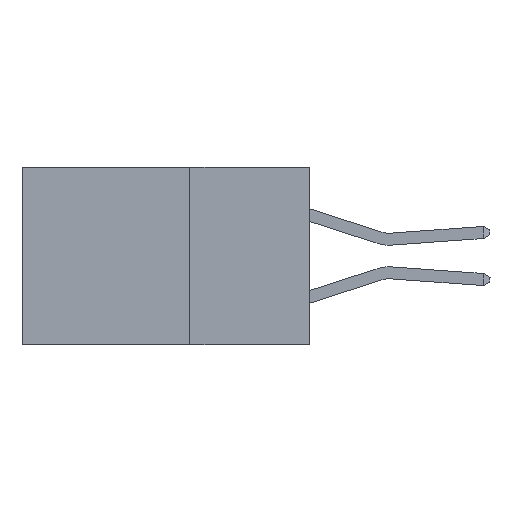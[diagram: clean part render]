
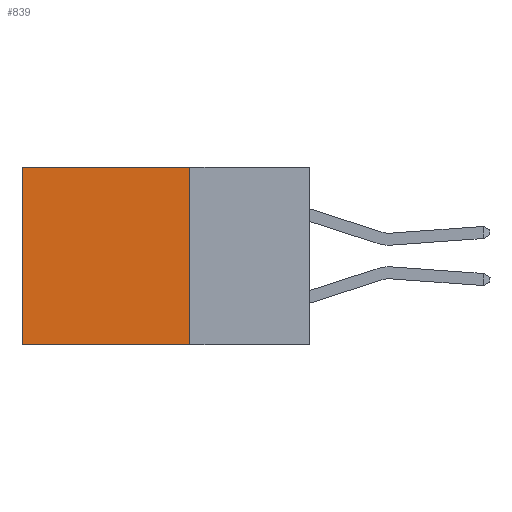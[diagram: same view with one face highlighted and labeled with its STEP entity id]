
A CAD part, left-side view. The second image highlights one B-rep face of the part: STEP entity #839.
In plain terms, the highlighted planar face has unit normal (-1, 0, 0).
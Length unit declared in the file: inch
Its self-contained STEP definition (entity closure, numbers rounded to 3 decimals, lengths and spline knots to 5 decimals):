
#684 = LINE ( 'NONE', #10776, #11433 ) ;
#839 = ADVANCED_FACE ( 'NONE', ( #4404 ), #17159, .F. ) ;
#1855 = DIRECTION ( 'NONE',  ( 0., 0., -1. ) ) ;
#2136 = ORIENTED_EDGE ( 'NONE', *, *, #6827, .F. ) ;
#3057 = CARTESIAN_POINT ( 'NONE',  ( 0.298, 0.25, 0. ) ) ;
#3497 = LINE ( 'NONE', #5003, #14112 ) ;
#4029 = ORIENTED_EDGE ( 'NONE', *, *, #14967, .T. ) ;
#4404 = FACE_OUTER_BOUND ( 'NONE', #16110, .T. ) ;
#4791 = EDGE_CURVE ( 'NONE', #10308, #5745, #684, .T. ) ;
#5003 = CARTESIAN_POINT ( 'NONE',  ( 0.298, 0.25, -0.37 ) ) ;
#5745 = VERTEX_POINT ( 'NONE', #11351 ) ;
#6730 = DIRECTION ( 'NONE',  ( 1., 0., 0. ) ) ;
#6827 = EDGE_CURVE ( 'NONE', #12102, #9563, #7291, .T. ) ;
#7291 = LINE ( 'NONE', #13268, #10555 ) ;
#7435 = ORIENTED_EDGE ( 'NONE', *, *, #12868, .F. ) ;
#9563 = VERTEX_POINT ( 'NONE', #14047 ) ;
#10053 = CARTESIAN_POINT ( 'NONE',  ( 0.298, 0.25, 0. ) ) ;
#10308 = VERTEX_POINT ( 'NONE', #13098 ) ;
#10555 = VECTOR ( 'NONE', #17623, 39.37008 ) ;
#10776 = CARTESIAN_POINT ( 'NONE',  ( 0.298, 0.6, 0. ) ) ;
#11351 = CARTESIAN_POINT ( 'NONE',  ( 0.298, 0.6, -0.37 ) ) ;
#11433 = VECTOR ( 'NONE', #13922, 39.37008 ) ;
#11852 = DIRECTION ( 'NONE',  ( 0., 1., 0. ) ) ;
#12102 = VERTEX_POINT ( 'NONE', #10053 ) ;
#12868 = EDGE_CURVE ( 'NONE', #9563, #5745, #3497, .T. ) ;
#13098 = CARTESIAN_POINT ( 'NONE',  ( 0.298, 0.6, 0. ) ) ;
#13268 = CARTESIAN_POINT ( 'NONE',  ( 0.298, 0.25, 0. ) ) ;
#13911 = ORIENTED_EDGE ( 'NONE', *, *, #4791, .T. ) ;
#13922 = DIRECTION ( 'NONE',  ( 0., 0., -1. ) ) ;
#14047 = CARTESIAN_POINT ( 'NONE',  ( 0.298, 0.25, -0.37 ) ) ;
#14112 = VECTOR ( 'NONE', #11852, 39.37008 ) ;
#14139 = DIRECTION ( 'NONE',  ( 0., 1., 0. ) ) ;
#14749 = AXIS2_PLACEMENT_3D ( 'NONE', #14963, #6730, #1855 ) ;
#14963 = CARTESIAN_POINT ( 'NONE',  ( 0.298, 0.25, 0. ) ) ;
#14967 = EDGE_CURVE ( 'NONE', #12102, #10308, #15712, .T. ) ;
#15712 = LINE ( 'NONE', #3057, #16117 ) ;
#16110 = EDGE_LOOP ( 'NONE', ( #13911, #7435, #2136, #4029 ) ) ;
#16117 = VECTOR ( 'NONE', #14139, 39.37008 ) ;
#17159 = PLANE ( 'NONE',  #14749 ) ;
#17623 = DIRECTION ( 'NONE',  ( 0., 0., -1. ) ) ;
